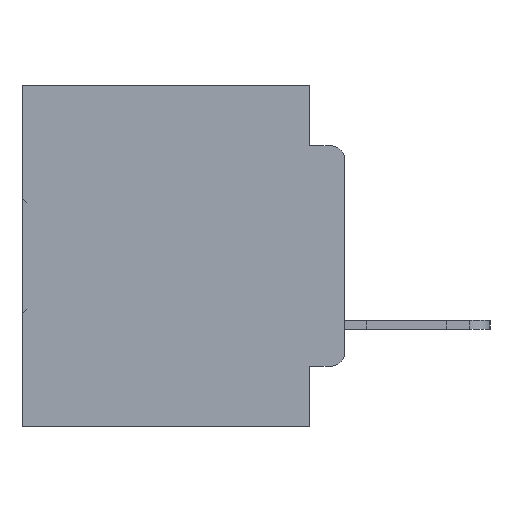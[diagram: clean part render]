
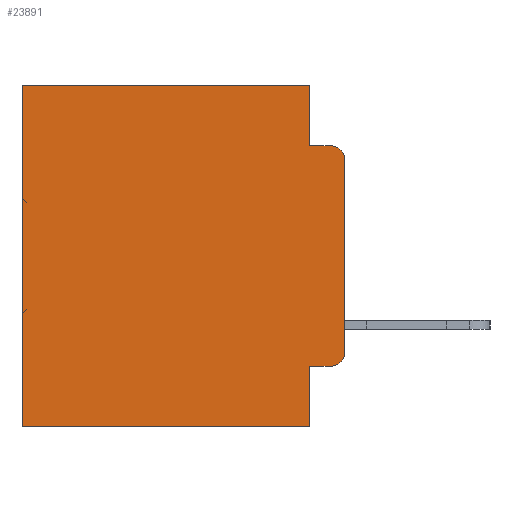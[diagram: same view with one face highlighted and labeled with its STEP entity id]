
A CAD part, left-side view. The second image highlights one B-rep face of the part: STEP entity #23891.
In plain terms, the highlighted planar face has unit normal (-1, 0, 0).
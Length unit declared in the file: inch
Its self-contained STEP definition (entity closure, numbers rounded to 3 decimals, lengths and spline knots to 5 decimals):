
#75 = VERTEX_POINT ( 'NONE', #11673 ) ;
#604 = VECTOR ( 'NONE', #10386, 39.37008 ) ;
#736 = DIRECTION ( 'NONE',  ( 0., 1., 0. ) ) ;
#1042 = DIRECTION ( 'NONE',  ( 0., 0., -1. ) ) ;
#2148 = CARTESIAN_POINT ( 'NONE',  ( 0.298, 0., -0.3915 ) ) ;
#2714 = VERTEX_POINT ( 'NONE', #25924 ) ;
#2872 = CARTESIAN_POINT ( 'NONE',  ( 0.298, 0., -0.1085 ) ) ;
#3095 = VECTOR ( 'NONE', #23323, 39.37008 ) ;
#4217 = EDGE_CURVE ( 'NONE', #17997, #13092, #5323, .T. ) ;
#4226 = CARTESIAN_POINT ( 'NONE',  ( 0.298, 0.051, -0.0885 ) ) ;
#5323 = LINE ( 'NONE', #30110, #3095 ) ;
#6636 = CIRCLE ( 'NONE', #19257, 0.02 ) ;
#7157 = LINE ( 'NONE', #27631, #22076 ) ;
#7287 = VECTOR ( 'NONE', #14517, 39.37008 ) ;
#7404 = LINE ( 'NONE', #34117, #28370 ) ;
#7776 = DIRECTION ( 'NONE',  ( 0., 0., -1. ) ) ;
#8239 = LINE ( 'NONE', #33498, #29129 ) ;
#8299 = CARTESIAN_POINT ( 'NONE',  ( 0.298, 0.051, 0. ) ) ;
#8366 = LINE ( 'NONE', #10838, #604 ) ;
#8801 = DIRECTION ( 'NONE',  ( 0., 0., -1. ) ) ;
#8829 = CIRCLE ( 'NONE', #12120, 0.02 ) ;
#8936 = VECTOR ( 'NONE', #736, 39.37008 ) ;
#9891 = LINE ( 'NONE', #24188, #8936 ) ;
#10258 = CARTESIAN_POINT ( 'NONE',  ( 0.298, 0.051, -0.5 ) ) ;
#10386 = DIRECTION ( 'NONE',  ( 0., -1., 0. ) ) ;
#10838 = CARTESIAN_POINT ( 'NONE',  ( 0.298, 0.051, -0.4115 ) ) ;
#11641 = VERTEX_POINT ( 'NONE', #10258 ) ;
#11673 = CARTESIAN_POINT ( 'NONE',  ( 0.298, 0.473, -0.5 ) ) ;
#12120 = AXIS2_PLACEMENT_3D ( 'NONE', #27873, #27111, #7776 ) ;
#12473 = VERTEX_POINT ( 'NONE', #30864 ) ;
#13092 = VERTEX_POINT ( 'NONE', #32455 ) ;
#13282 = CARTESIAN_POINT ( 'NONE',  ( 0.298, 0.051, 0. ) ) ;
#13485 = FACE_OUTER_BOUND ( 'NONE', #19792, .T. ) ;
#14517 = DIRECTION ( 'NONE',  ( 0., -1., 0. ) ) ;
#15072 = LINE ( 'NONE', #35147, #7287 ) ;
#15321 = EDGE_CURVE ( 'NONE', #12473, #11641, #8239, .T. ) ;
#15383 = VERTEX_POINT ( 'NONE', #2148 ) ;
#15795 = EDGE_CURVE ( 'NONE', #30867, #2714, #15072, .T. ) ;
#16196 = ORIENTED_EDGE ( 'NONE', *, *, #24255, .T. ) ;
#16541 = ORIENTED_EDGE ( 'NONE', *, *, #17611, .F. ) ;
#16978 = ORIENTED_EDGE ( 'NONE', *, *, #18035, .F. ) ;
#17611 = EDGE_CURVE ( 'NONE', #28667, #15383, #7157, .T. ) ;
#17997 = VERTEX_POINT ( 'NONE', #8299 ) ;
#18035 = EDGE_CURVE ( 'NONE', #11641, #75, #9891, .T. ) ;
#18097 = VECTOR ( 'NONE', #23850, 39.37008 ) ;
#18288 = DIRECTION ( 'NONE',  ( -1., 0., 0. ) ) ;
#18776 = CARTESIAN_POINT ( 'NONE',  ( 0.298, 0.02, -0.4115 ) ) ;
#19257 = AXIS2_PLACEMENT_3D ( 'NONE', #33951, #18288, #1042 ) ;
#19792 = EDGE_LOOP ( 'NONE', ( #16541, #24437, #26523, #30203, #23140, #29717, #16978, #29570, #16196, #32471 ) ) ;
#20169 = AXIS2_PLACEMENT_3D ( 'NONE', #27241, #22160, #29092 ) ;
#22076 = VECTOR ( 'NONE', #35149, 39.37008 ) ;
#22160 = DIRECTION ( 'NONE',  ( 1., 0., 0. ) ) ;
#22386 = PLANE ( 'NONE',  #20169 ) ;
#23140 = ORIENTED_EDGE ( 'NONE', *, *, #4217, .T. ) ;
#23323 = DIRECTION ( 'NONE',  ( 0., 1., 0. ) ) ;
#23850 = DIRECTION ( 'NONE',  ( 0., 0., -1. ) ) ;
#23891 = ADVANCED_FACE ( 'NONE', ( #13485 ), #22386, .F. ) ;
#24188 = CARTESIAN_POINT ( 'NONE',  ( 0.298, 0., -0.5 ) ) ;
#24255 = EDGE_CURVE ( 'NONE', #12473, #24864, #8366, .T. ) ;
#24437 = ORIENTED_EDGE ( 'NONE', *, *, #33421, .T. ) ;
#24864 = VERTEX_POINT ( 'NONE', #18776 ) ;
#25135 = LINE ( 'NONE', #13282, #18097 ) ;
#25924 = CARTESIAN_POINT ( 'NONE',  ( 0.298, 0.02, -0.0885 ) ) ;
#26267 = DIRECTION ( 'NONE',  ( 0., 0., -1. ) ) ;
#26523 = ORIENTED_EDGE ( 'NONE', *, *, #15795, .F. ) ;
#26651 = EDGE_CURVE ( 'NONE', #24864, #15383, #8829, .T. ) ;
#27111 = DIRECTION ( 'NONE',  ( -1., 0., 0. ) ) ;
#27241 = CARTESIAN_POINT ( 'NONE',  ( 0.298, 0., 0. ) ) ;
#27631 = CARTESIAN_POINT ( 'NONE',  ( 0.298, 0., 0. ) ) ;
#27873 = CARTESIAN_POINT ( 'NONE',  ( 0.298, 0.02, -0.3915 ) ) ;
#28370 = VECTOR ( 'NONE', #26267, 39.37008 ) ;
#28667 = VERTEX_POINT ( 'NONE', #2872 ) ;
#28796 = EDGE_CURVE ( 'NONE', #17997, #30867, #25135, .T. ) ;
#29092 = DIRECTION ( 'NONE',  ( 0., 0., -1. ) ) ;
#29129 = VECTOR ( 'NONE', #8801, 39.37008 ) ;
#29570 = ORIENTED_EDGE ( 'NONE', *, *, #15321, .F. ) ;
#29717 = ORIENTED_EDGE ( 'NONE', *, *, #34718, .T. ) ;
#30110 = CARTESIAN_POINT ( 'NONE',  ( 0.298, 0., 0. ) ) ;
#30203 = ORIENTED_EDGE ( 'NONE', *, *, #28796, .F. ) ;
#30864 = CARTESIAN_POINT ( 'NONE',  ( 0.298, 0.051, -0.4115 ) ) ;
#30867 = VERTEX_POINT ( 'NONE', #4226 ) ;
#32455 = CARTESIAN_POINT ( 'NONE',  ( 0.298, 0.473, 0. ) ) ;
#32471 = ORIENTED_EDGE ( 'NONE', *, *, #26651, .T. ) ;
#33421 = EDGE_CURVE ( 'NONE', #28667, #2714, #6636, .T. ) ;
#33498 = CARTESIAN_POINT ( 'NONE',  ( 0.298, 0.051, 0. ) ) ;
#33951 = CARTESIAN_POINT ( 'NONE',  ( 0.298, 0.02, -0.1085 ) ) ;
#34117 = CARTESIAN_POINT ( 'NONE',  ( 0.298, 0.473, 0. ) ) ;
#34718 = EDGE_CURVE ( 'NONE', #13092, #75, #7404, .T. ) ;
#35147 = CARTESIAN_POINT ( 'NONE',  ( 0.298, 0.051, -0.0885 ) ) ;
#35149 = DIRECTION ( 'NONE',  ( 0., 0., -1. ) ) ;
